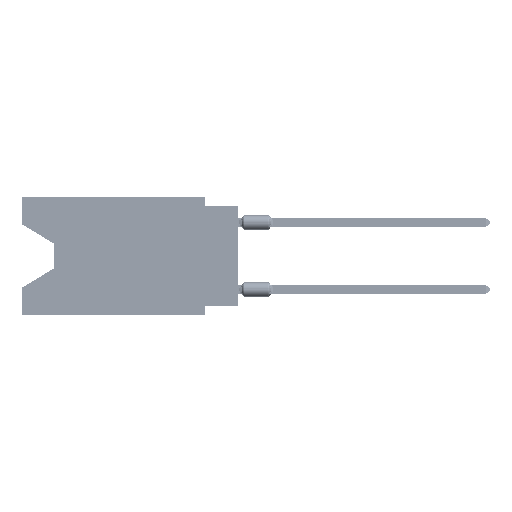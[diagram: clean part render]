
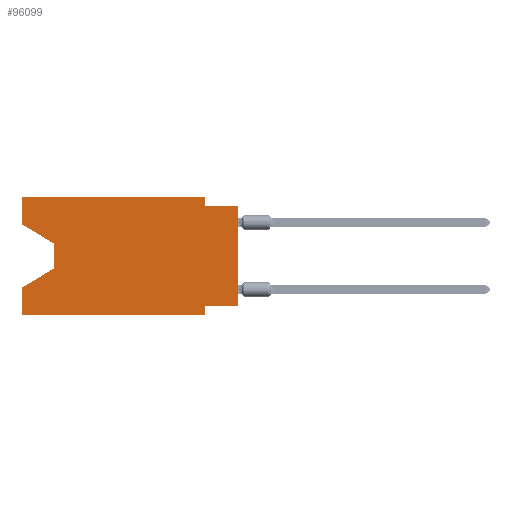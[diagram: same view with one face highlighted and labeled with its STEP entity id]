
A CAD part, left-side view. The second image highlights one B-rep face of the part: STEP entity #96099.
In plain terms, the highlighted planar face has unit normal (-1, 0, 0).
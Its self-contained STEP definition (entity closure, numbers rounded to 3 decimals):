
#38 = ORIENTED_EDGE ( 'NONE', *, *, #36947, .T. ) ;
#766 = EDGE_CURVE ( 'NONE', #8824, #37604, #89019, .T. ) ;
#1164 = AXIS2_PLACEMENT_3D ( 'NONE', #80819, #55010, #105540 ) ;
#1911 = EDGE_CURVE ( 'NONE', #37604, #19807, #86819, .T. ) ;
#3552 = EDGE_CURVE ( 'NONE', #30392, #67086, #93974, .T. ) ;
#5208 = CARTESIAN_POINT ( 'NONE',  ( 0., 2.54, -8.255 ) ) ;
#8163 = LINE ( 'NONE', #42382, #10517 ) ;
#8824 = VERTEX_POINT ( 'NONE', #106299 ) ;
#8918 = VERTEX_POINT ( 'NONE', #75923 ) ;
#10517 = VECTOR ( 'NONE', #42941, 1000. ) ;
#11445 = DIRECTION ( 'NONE',  ( 0., 0., 1. ) ) ;
#12001 = CARTESIAN_POINT ( 'NONE',  ( 0., 16.383, 0. ) ) ;
#12436 = EDGE_CURVE ( 'NONE', #103211, #84619, #21910, .T. ) ;
#12484 = VECTOR ( 'NONE', #46024, 1000. ) ;
#12617 = CARTESIAN_POINT ( 'NONE',  ( 0., 16.383, -6.852 ) ) ;
#13743 = EDGE_CURVE ( 'NONE', #22085, #8918, #75769, .T. ) ;
#14092 = VECTOR ( 'NONE', #41528, 1000. ) ;
#14913 = EDGE_CURVE ( 'NONE', #84619, #22190, #54438, .T. ) ;
#19118 = CARTESIAN_POINT ( 'NONE',  ( 0., 13.97, -5.385 ) ) ;
#19807 = VERTEX_POINT ( 'NONE', #54042 ) ;
#21197 = VECTOR ( 'NONE', #97139, 1000. ) ;
#21303 = LINE ( 'NONE', #30282, #91472 ) ;
#21910 = LINE ( 'NONE', #56139, #42346 ) ;
#22085 = VERTEX_POINT ( 'NONE', #22895 ) ;
#22190 = VERTEX_POINT ( 'NONE', #12617 ) ;
#22895 = CARTESIAN_POINT ( 'NONE',  ( 0., 0., -8.255 ) ) ;
#22965 = VECTOR ( 'NONE', #70336, 1000. ) ;
#23156 = VECTOR ( 'NONE', #25507, 1000. ) ;
#23369 = CARTESIAN_POINT ( 'NONE',  ( 0., 2.54, -0.635 ) ) ;
#25507 = DIRECTION ( 'NONE',  ( 0., -1., 0. ) ) ;
#30282 = CARTESIAN_POINT ( 'NONE',  ( 0., 2.54, 0. ) ) ;
#30392 = VERTEX_POINT ( 'NONE', #43737 ) ;
#34480 = CARTESIAN_POINT ( 'NONE',  ( 0., 16.383, -8.89 ) ) ;
#34679 = VERTEX_POINT ( 'NONE', #23369 ) ;
#36485 = EDGE_CURVE ( 'NONE', #97294, #67086, #94534, .T. ) ;
#36947 = EDGE_CURVE ( 'NONE', #8824, #103211, #89281, .T. ) ;
#37604 = VERTEX_POINT ( 'NONE', #100314 ) ;
#39206 = ORIENTED_EDGE ( 'NONE', *, *, #90757, .F. ) ;
#40180 = LINE ( 'NONE', #89622, #100669 ) ;
#41528 = DIRECTION ( 'NONE',  ( 0., 0., 1. ) ) ;
#42075 = CARTESIAN_POINT ( 'NONE',  ( 0., 0., 0. ) ) ;
#42346 = VECTOR ( 'NONE', #79188, 1000. ) ;
#42382 = CARTESIAN_POINT ( 'NONE',  ( 0., 0., -0.635 ) ) ;
#42941 = DIRECTION ( 'NONE',  ( 0., -1., 0. ) ) ;
#43737 = CARTESIAN_POINT ( 'NONE',  ( 0., 16.383, -8.89 ) ) ;
#46024 = DIRECTION ( 'NONE',  ( 0., 0.855, -0.519 ) ) ;
#46074 = VECTOR ( 'NONE', #63194, 1000. ) ;
#46240 = VECTOR ( 'NONE', #46370, 1000. ) ;
#46370 = DIRECTION ( 'NONE',  ( 0., -1., 0. ) ) ;
#51851 = CARTESIAN_POINT ( 'NONE',  ( 0., 2.54, -8.89 ) ) ;
#54042 = CARTESIAN_POINT ( 'NONE',  ( 0., 2.54, 0. ) ) ;
#54079 = LINE ( 'NONE', #12001, #105554 ) ;
#54438 = LINE ( 'NONE', #19118, #12484 ) ;
#54588 = CARTESIAN_POINT ( 'NONE',  ( 0., 13.97, -3.505 ) ) ;
#55010 = DIRECTION ( 'NONE',  ( 1., 0., 0. ) ) ;
#55073 = ORIENTED_EDGE ( 'NONE', *, *, #12436, .T. ) ;
#56139 = CARTESIAN_POINT ( 'NONE',  ( 0., 13.97, -3.505 ) ) ;
#60670 = ORIENTED_EDGE ( 'NONE', *, *, #766, .F. ) ;
#61540 = CARTESIAN_POINT ( 'NONE',  ( 0., 16.383, 0. ) ) ;
#62902 = CARTESIAN_POINT ( 'NONE',  ( 0., 16.383, -2.038 ) ) ;
#63194 = DIRECTION ( 'NONE',  ( 0., 0., 1. ) ) ;
#64279 = EDGE_LOOP ( 'NONE', ( #38, #55073, #74166, #109263, #80491, #71908, #78720, #71493, #39206, #80519, #86822, #60670 ) ) ;
#64513 = DIRECTION ( 'NONE',  ( 0., 0., -1. ) ) ;
#65475 = EDGE_CURVE ( 'NONE', #19807, #34679, #21303, .T. ) ;
#67086 = VERTEX_POINT ( 'NONE', #105902 ) ;
#67296 = EDGE_CURVE ( 'NONE', #22085, #97294, #40180, .T. ) ;
#69060 = CARTESIAN_POINT ( 'NONE',  ( 0., 13.97, -5.385 ) ) ;
#70336 = DIRECTION ( 'NONE',  ( 0., 0., -1. ) ) ;
#71285 = PLANE ( 'NONE',  #1164 ) ;
#71493 = ORIENTED_EDGE ( 'NONE', *, *, #13743, .T. ) ;
#71908 = ORIENTED_EDGE ( 'NONE', *, *, #36485, .F. ) ;
#74166 = ORIENTED_EDGE ( 'NONE', *, *, #14913, .T. ) ;
#75769 = LINE ( 'NONE', #42075, #14092 ) ;
#75923 = CARTESIAN_POINT ( 'NONE',  ( 0., 0., -0.635 ) ) ;
#78720 = ORIENTED_EDGE ( 'NONE', *, *, #67296, .F. ) ;
#79188 = DIRECTION ( 'NONE',  ( 0., 0., -1. ) ) ;
#80491 = ORIENTED_EDGE ( 'NONE', *, *, #3552, .T. ) ;
#80519 = ORIENTED_EDGE ( 'NONE', *, *, #65475, .F. ) ;
#80819 = CARTESIAN_POINT ( 'NONE',  ( 0., 16.383, 0. ) ) ;
#84619 = VERTEX_POINT ( 'NONE', #69060 ) ;
#86819 = LINE ( 'NONE', #88480, #46240 ) ;
#86822 = ORIENTED_EDGE ( 'NONE', *, *, #1911, .F. ) ;
#88480 = CARTESIAN_POINT ( 'NONE',  ( 0., 16.383, 0. ) ) ;
#89019 = LINE ( 'NONE', #61540, #46074 ) ;
#89281 = LINE ( 'NONE', #62902, #21197 ) ;
#89622 = CARTESIAN_POINT ( 'NONE',  ( 0., 0., -8.255 ) ) ;
#90757 = EDGE_CURVE ( 'NONE', #34679, #8918, #8163, .T. ) ;
#91472 = VECTOR ( 'NONE', #64513, 1000. ) ;
#93974 = LINE ( 'NONE', #34480, #23156 ) ;
#94534 = LINE ( 'NONE', #51851, #22965 ) ;
#96099 = ADVANCED_FACE ( 'NONE', ( #97670 ), #71285, .F. ) ;
#97139 = DIRECTION ( 'NONE',  ( 0., -0.855, -0.519 ) ) ;
#97294 = VERTEX_POINT ( 'NONE', #5208 ) ;
#97670 = FACE_OUTER_BOUND ( 'NONE', #64279, .T. ) ;
#98582 = DIRECTION ( 'NONE',  ( 0., 1., 0. ) ) ;
#99227 = EDGE_CURVE ( 'NONE', #30392, #22190, #54079, .T. ) ;
#100314 = CARTESIAN_POINT ( 'NONE',  ( 0., 16.383, 0. ) ) ;
#100669 = VECTOR ( 'NONE', #98582, 1000. ) ;
#103211 = VERTEX_POINT ( 'NONE', #54588 ) ;
#105540 = DIRECTION ( 'NONE',  ( 0., 0., -1. ) ) ;
#105554 = VECTOR ( 'NONE', #11445, 1000. ) ;
#105902 = CARTESIAN_POINT ( 'NONE',  ( 0., 2.54, -8.89 ) ) ;
#106299 = CARTESIAN_POINT ( 'NONE',  ( 0., 16.383, -2.038 ) ) ;
#109263 = ORIENTED_EDGE ( 'NONE', *, *, #99227, .F. ) ;
